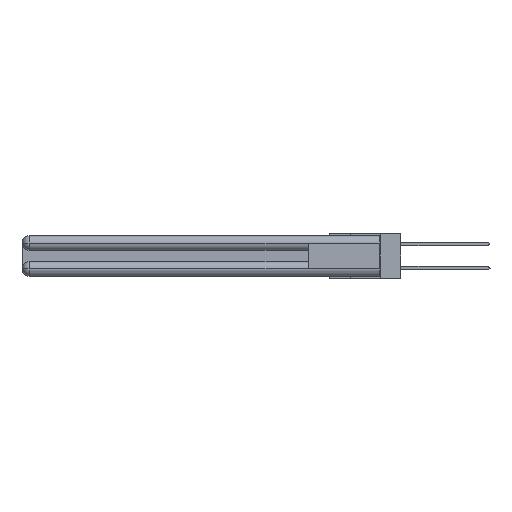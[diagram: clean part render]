
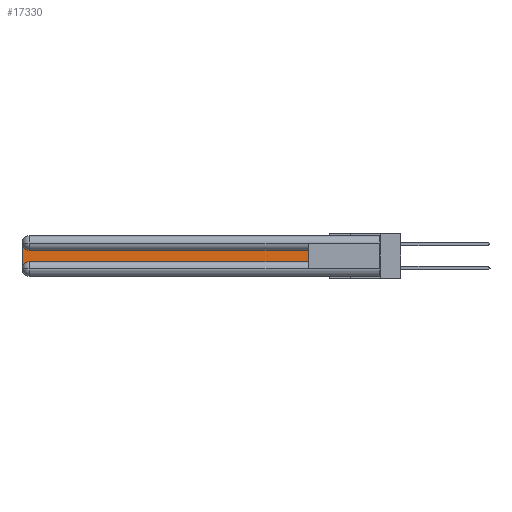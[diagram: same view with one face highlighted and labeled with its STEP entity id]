
A CAD part, left-side view. The second image highlights one B-rep face of the part: STEP entity #17330.
In plain terms, the highlighted planar face has unit normal (-1, 0, 0).
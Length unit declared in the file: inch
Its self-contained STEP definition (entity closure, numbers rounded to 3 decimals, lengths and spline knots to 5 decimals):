
#97 = ORIENTED_EDGE ( 'NONE', *, *, #35273, .T. ) ;
#108 = DIRECTION ( 'NONE',  ( 0., 0., -1. ) ) ;
#687 = VECTOR ( 'NONE', #31267, 39.37008 ) ;
#2117 = DIRECTION ( 'NONE',  ( 1., 0., 0. ) ) ;
#2359 = CARTESIAN_POINT ( 'NONE',  ( 0.075, 3., -0.2775 ) ) ;
#2838 = LINE ( 'NONE', #19586, #13648 ) ;
#2854 = CARTESIAN_POINT ( 'NONE',  ( 0.075, 0.6, -0.2175 ) ) ;
#3151 = LINE ( 'NONE', #32458, #35147 ) ;
#4546 = LINE ( 'NONE', #6332, #687 ) ;
#5527 = ORIENTED_EDGE ( 'NONE', *, *, #17026, .T. ) ;
#6332 = CARTESIAN_POINT ( 'NONE',  ( 0.075, 0.6, -0.2175 ) ) ;
#7396 = ORIENTED_EDGE ( 'NONE', *, *, #24544, .T. ) ;
#7844 = VERTEX_POINT ( 'NONE', #25315 ) ;
#8502 = ORIENTED_EDGE ( 'NONE', *, *, #14100, .T. ) ;
#8658 = AXIS2_PLACEMENT_3D ( 'NONE', #30105, #10368, #13650 ) ;
#10368 = DIRECTION ( 'NONE',  ( 1., 0., 0. ) ) ;
#12401 = VERTEX_POINT ( 'NONE', #15569 ) ;
#12976 = CARTESIAN_POINT ( 'NONE',  ( 0.075, 2.94, -0.0625 ) ) ;
#13424 = VERTEX_POINT ( 'NONE', #2359 ) ;
#13648 = VECTOR ( 'NONE', #108, 39.37008 ) ;
#13650 = DIRECTION ( 'NONE',  ( 0., 0., -1. ) ) ;
#14100 = EDGE_CURVE ( 'NONE', #20719, #31633, #3151, .T. ) ;
#15569 = CARTESIAN_POINT ( 'NONE',  ( 0.075, 3., -0.0625 ) ) ;
#15582 = EDGE_LOOP ( 'NONE', ( #8502, #97, #7396, #26493, #29862, #5527 ) ) ;
#15626 = DIRECTION ( 'NONE',  ( 0., 0., -1. ) ) ;
#15975 = DIRECTION ( 'NONE',  ( 0., 1., 0. ) ) ;
#16342 = DIRECTION ( 'NONE',  ( 1., 0., 0. ) ) ;
#16483 = DIRECTION ( 'NONE',  ( 0., -1., 0. ) ) ;
#17026 = EDGE_CURVE ( 'NONE', #18983, #20719, #4546, .T. ) ;
#17330 = ADVANCED_FACE ( 'NONE', ( #26179 ), #21407, .F. ) ;
#18983 = VERTEX_POINT ( 'NONE', #2854 ) ;
#19177 = CARTESIAN_POINT ( 'NONE',  ( 0.075, 2.94, -0.1225 ) ) ;
#19286 = DIRECTION ( 'NONE',  ( 0., 0., -1. ) ) ;
#19432 = AXIS2_PLACEMENT_3D ( 'NONE', #30268, #16342, #19286 ) ;
#19586 = CARTESIAN_POINT ( 'NONE',  ( 0.075, 3., -0.2175 ) ) ;
#20719 = VERTEX_POINT ( 'NONE', #29041 ) ;
#21407 = PLANE ( 'NONE',  #8658 ) ;
#22043 = EDGE_CURVE ( 'NONE', #13424, #7844, #26311, .T. ) ;
#23014 = CIRCLE ( 'NONE', #32208, 0.06 ) ;
#24038 = LINE ( 'NONE', #34402, #25761 ) ;
#24544 = EDGE_CURVE ( 'NONE', #12401, #13424, #2838, .T. ) ;
#25315 = CARTESIAN_POINT ( 'NONE',  ( 0.075, 2.94, -0.2175 ) ) ;
#25761 = VECTOR ( 'NONE', #16483, 39.37008 ) ;
#26179 = FACE_OUTER_BOUND ( 'NONE', #15582, .T. ) ;
#26311 = CIRCLE ( 'NONE', #19432, 0.06 ) ;
#26493 = ORIENTED_EDGE ( 'NONE', *, *, #22043, .T. ) ;
#29041 = CARTESIAN_POINT ( 'NONE',  ( 0.075, 0.6, -0.1225 ) ) ;
#29862 = ORIENTED_EDGE ( 'NONE', *, *, #31604, .T. ) ;
#30105 = CARTESIAN_POINT ( 'NONE',  ( 0.075, 3., -0.1225 ) ) ;
#30268 = CARTESIAN_POINT ( 'NONE',  ( 0.075, 2.94, -0.2775 ) ) ;
#31267 = DIRECTION ( 'NONE',  ( 0., 0., 1. ) ) ;
#31604 = EDGE_CURVE ( 'NONE', #7844, #18983, #24038, .T. ) ;
#31633 = VERTEX_POINT ( 'NONE', #19177 ) ;
#32208 = AXIS2_PLACEMENT_3D ( 'NONE', #12976, #2117, #15626 ) ;
#32458 = CARTESIAN_POINT ( 'NONE',  ( 0.075, 0.6, -0.1225 ) ) ;
#34402 = CARTESIAN_POINT ( 'NONE',  ( 0.075, 0.6, -0.2175 ) ) ;
#35147 = VECTOR ( 'NONE', #15975, 39.37008 ) ;
#35273 = EDGE_CURVE ( 'NONE', #31633, #12401, #23014, .T. ) ;
